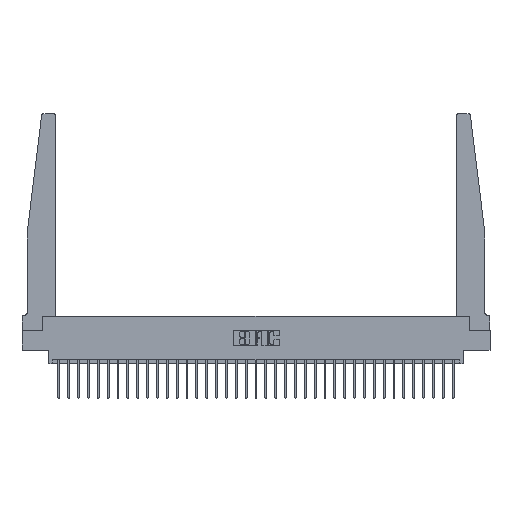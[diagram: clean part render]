
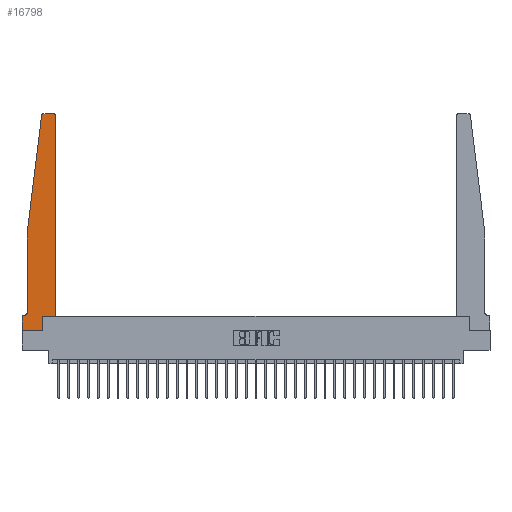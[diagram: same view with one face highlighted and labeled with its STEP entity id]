
A CAD part, top view. The second image highlights one B-rep face of the part: STEP entity #16798.
In plain terms, the highlighted planar face has unit normal (0, 0, 1).
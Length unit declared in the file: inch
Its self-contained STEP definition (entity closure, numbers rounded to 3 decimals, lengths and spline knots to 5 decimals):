
#13 = CARTESIAN_POINT ( 'NONE',  ( 0., 0.1875, 0.37 ) ) ;
#253 = DIRECTION ( 'NONE',  ( 0., 1., 0. ) ) ;
#293 = EDGE_CURVE ( 'NONE', #13988, #8961, #5187, .T. ) ;
#1033 = VERTEX_POINT ( 'NONE', #15964 ) ;
#1728 = DIRECTION ( 'NONE',  ( 1., 0., 0. ) ) ;
#1989 = VECTOR ( 'NONE', #6766, 39.37008 ) ;
#2182 = CARTESIAN_POINT ( 'NONE',  ( 0.065, 1.25, 0.37 ) ) ;
#2205 = DIRECTION ( 'NONE',  ( 1., 0., 0. ) ) ;
#2500 = DIRECTION ( 'NONE',  ( 1., 0., 0. ) ) ;
#3809 = CARTESIAN_POINT ( 'NONE',  ( 0.27653, 2.75, 0.37 ) ) ;
#3878 = VECTOR ( 'NONE', #24932, 39.37008 ) ;
#3992 = EDGE_CURVE ( 'NONE', #31811, #25784, #8619, .T. ) ;
#4473 = LINE ( 'NONE', #31294, #29850 ) ;
#4556 = AXIS2_PLACEMENT_3D ( 'NONE', #9377, #26571, #11857 ) ;
#4773 = VECTOR ( 'NONE', #10022, 39.37008 ) ;
#5178 = VECTOR ( 'NONE', #16942, 39.37008 ) ;
#5187 = CIRCLE ( 'NONE', #25528, 0.05 ) ;
#5251 = CARTESIAN_POINT ( 'NONE',  ( 0.065, 1.25, 0.37 ) ) ;
#6358 = LINE ( 'NONE', #23235, #25223 ) ;
#6387 = ORIENTED_EDGE ( 'NONE', *, *, #9604, .T. ) ;
#6766 = DIRECTION ( 'NONE',  ( -1., 0., 0. ) ) ;
#7552 = CARTESIAN_POINT ( 'NONE',  ( 0.425, 0.18, 0.37 ) ) ;
#8388 = AXIS2_PLACEMENT_3D ( 'NONE', #31647, #16973, #2205 ) ;
#8418 = CIRCLE ( 'NONE', #8388, 0.03 ) ;
#8619 = LINE ( 'NONE', #14095, #1989 ) ;
#8897 = CARTESIAN_POINT ( 'NONE',  ( 0., 0., 0.37 ) ) ;
#8903 = EDGE_CURVE ( 'NONE', #1033, #12579, #12298, .T. ) ;
#8961 = VERTEX_POINT ( 'NONE', #28784 ) ;
#9312 = ORIENTED_EDGE ( 'NONE', *, *, #16701, .T. ) ;
#9377 = CARTESIAN_POINT ( 'NONE',  ( 0.395, 2.72, 0.37 ) ) ;
#9412 = FACE_OUTER_BOUND ( 'NONE', #24516, .T. ) ;
#9604 = EDGE_CURVE ( 'NONE', #25784, #17146, #8418, .T. ) ;
#9636 = ORIENTED_EDGE ( 'NONE', *, *, #29776, .T. ) ;
#10022 = DIRECTION ( 'NONE',  ( 1., 0., 0. ) ) ;
#10501 = LINE ( 'NONE', #5251, #3878 ) ;
#11056 = ORIENTED_EDGE ( 'NONE', *, *, #8903, .T. ) ;
#11343 = LINE ( 'NONE', #7552, #4773 ) ;
#11408 = DIRECTION ( 'NONE',  ( 0., 1., 0. ) ) ;
#11629 = DIRECTION ( 'NONE',  ( 0., 0., -1. ) ) ;
#11632 = VERTEX_POINT ( 'NONE', #14952 ) ;
#11674 = VECTOR ( 'NONE', #1728, 39.37008 ) ;
#11857 = DIRECTION ( 'NONE',  ( 1., 0., 0. ) ) ;
#11910 = ORIENTED_EDGE ( 'NONE', *, *, #29931, .T. ) ;
#12195 = ORIENTED_EDGE ( 'NONE', *, *, #3992, .T. ) ;
#12298 = LINE ( 'NONE', #28564, #24589 ) ;
#12355 = PLANE ( 'NONE',  #17533 ) ;
#12579 = VERTEX_POINT ( 'NONE', #29212 ) ;
#13137 = EDGE_CURVE ( 'NONE', #17146, #30983, #10501, .T. ) ;
#13294 = ORIENTED_EDGE ( 'NONE', *, *, #31370, .T. ) ;
#13468 = CARTESIAN_POINT ( 'NONE',  ( 0.065, 1.25, 0.37 ) ) ;
#13988 = VERTEX_POINT ( 'NONE', #23039 ) ;
#14095 = CARTESIAN_POINT ( 'NONE',  ( 0.25, 2.75, 0.37 ) ) ;
#14269 = DIRECTION ( 'NONE',  ( -1., 0., 0. ) ) ;
#14952 = CARTESIAN_POINT ( 'NONE',  ( 0., 0.1875, 0.37 ) ) ;
#15236 = EDGE_CURVE ( 'NONE', #8961, #11632, #4473, .T. ) ;
#15578 = CARTESIAN_POINT ( 'NONE',  ( 0., 0., 0.37 ) ) ;
#15964 = CARTESIAN_POINT ( 'NONE',  ( 0.425, 0.18, 0.37 ) ) ;
#16399 = EDGE_CURVE ( 'NONE', #11632, #23215, #6358, .T. ) ;
#16701 = EDGE_CURVE ( 'NONE', #30983, #13988, #24030, .T. ) ;
#16798 = ADVANCED_FACE ( 'NONE', ( #9412 ), #12355, .T. ) ;
#16942 = DIRECTION ( 'NONE',  ( 0., -1., 0. ) ) ;
#16973 = DIRECTION ( 'NONE',  ( 0., 0., 1. ) ) ;
#17146 = VERTEX_POINT ( 'NONE', #18959 ) ;
#17262 = DIRECTION ( 'NONE',  ( 0., 0., 1. ) ) ;
#17338 = ORIENTED_EDGE ( 'NONE', *, *, #15236, .T. ) ;
#17533 = AXIS2_PLACEMENT_3D ( 'NONE', #13, #17262, #2500 ) ;
#17755 = VECTOR ( 'NONE', #253, 39.37008 ) ;
#18193 = LINE ( 'NONE', #8897, #11674 ) ;
#18511 = LINE ( 'NONE', #24832, #17755 ) ;
#18959 = CARTESIAN_POINT ( 'NONE',  ( 0.24675, 2.72367, 0.37 ) ) ;
#19317 = VERTEX_POINT ( 'NONE', #26495 ) ;
#20954 = ORIENTED_EDGE ( 'NONE', *, *, #16399, .T. ) ;
#21172 = CARTESIAN_POINT ( 'NONE',  ( 0.2605, 0., 0.37 ) ) ;
#23039 = CARTESIAN_POINT ( 'NONE',  ( 0.065, 0.2375, 0.37 ) ) ;
#23215 = VERTEX_POINT ( 'NONE', #15578 ) ;
#23235 = CARTESIAN_POINT ( 'NONE',  ( 0., 0., 0.37 ) ) ;
#23440 = EDGE_CURVE ( 'NONE', #23215, #29644, #18193, .T. ) ;
#24030 = LINE ( 'NONE', #2182, #5178 ) ;
#24051 = CARTESIAN_POINT ( 'NONE',  ( 0.395, 2.75, 0.37 ) ) ;
#24516 = EDGE_LOOP ( 'NONE', ( #12195, #6387, #25040, #9312, #28725, #17338, #20954, #24664, #13294, #11910, #11056, #9636 ) ) ;
#24589 = VECTOR ( 'NONE', #11408, 39.37008 ) ;
#24664 = ORIENTED_EDGE ( 'NONE', *, *, #23440, .T. ) ;
#24832 = CARTESIAN_POINT ( 'NONE',  ( 0.2605, 0.18, 0.37 ) ) ;
#24932 = DIRECTION ( 'NONE',  ( -0.122, -0.992, 0. ) ) ;
#25040 = ORIENTED_EDGE ( 'NONE', *, *, #13137, .T. ) ;
#25223 = VECTOR ( 'NONE', #28146, 39.37008 ) ;
#25528 = AXIS2_PLACEMENT_3D ( 'NONE', #26489, #11629, #26347 ) ;
#25784 = VERTEX_POINT ( 'NONE', #3809 ) ;
#26347 = DIRECTION ( 'NONE',  ( -1., 0., 0. ) ) ;
#26489 = CARTESIAN_POINT ( 'NONE',  ( 0.015, 0.2375, 0.37 ) ) ;
#26495 = CARTESIAN_POINT ( 'NONE',  ( 0.2605, 0.18, 0.37 ) ) ;
#26571 = DIRECTION ( 'NONE',  ( 0., 0., 1. ) ) ;
#27500 = CIRCLE ( 'NONE', #4556, 0.03 ) ;
#28146 = DIRECTION ( 'NONE',  ( 0., -1., 0. ) ) ;
#28564 = CARTESIAN_POINT ( 'NONE',  ( 0.425, 0.18, 0.37 ) ) ;
#28725 = ORIENTED_EDGE ( 'NONE', *, *, #293, .T. ) ;
#28784 = CARTESIAN_POINT ( 'NONE',  ( 0.015, 0.1875, 0.37 ) ) ;
#29212 = CARTESIAN_POINT ( 'NONE',  ( 0.425, 2.72, 0.37 ) ) ;
#29644 = VERTEX_POINT ( 'NONE', #21172 ) ;
#29776 = EDGE_CURVE ( 'NONE', #12579, #31811, #27500, .T. ) ;
#29850 = VECTOR ( 'NONE', #14269, 39.37008 ) ;
#29931 = EDGE_CURVE ( 'NONE', #19317, #1033, #11343, .T. ) ;
#30983 = VERTEX_POINT ( 'NONE', #13468 ) ;
#31294 = CARTESIAN_POINT ( 'NONE',  ( 0.065, 0.1875, 0.37 ) ) ;
#31370 = EDGE_CURVE ( 'NONE', #29644, #19317, #18511, .T. ) ;
#31647 = CARTESIAN_POINT ( 'NONE',  ( 0.27653, 2.72, 0.37 ) ) ;
#31811 = VERTEX_POINT ( 'NONE', #24051 ) ;
